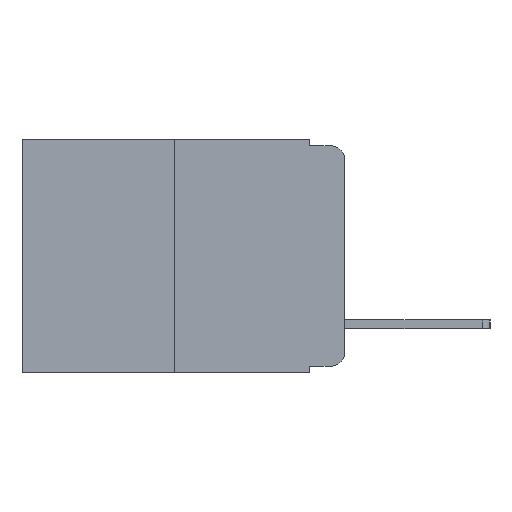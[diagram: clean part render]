
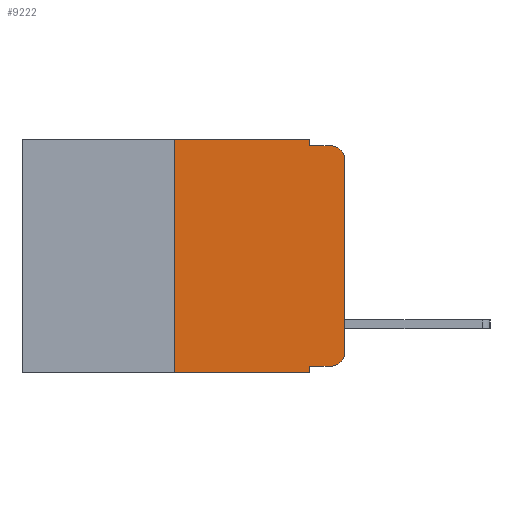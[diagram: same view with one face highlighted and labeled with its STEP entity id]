
A CAD part, left-side view. The second image highlights one B-rep face of the part: STEP entity #9222.
In plain terms, the highlighted planar face has unit normal (-1, 0, 0).
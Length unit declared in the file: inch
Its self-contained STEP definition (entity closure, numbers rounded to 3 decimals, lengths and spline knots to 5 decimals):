
#8 = VECTOR ( 'NONE', #17643, 39.37008 ) ;
#455 = AXIS2_PLACEMENT_3D ( 'NONE', #5341, #14909, #6776 ) ;
#684 = LINE ( 'NONE', #1124, #8795 ) ;
#1057 = CARTESIAN_POINT ( 'NONE',  ( 0., 0.25, -0.343 ) ) ;
#1124 = CARTESIAN_POINT ( 'NONE',  ( 0., 0.473, -0.343 ) ) ;
#1264 = LINE ( 'NONE', #2691, #8838 ) ;
#1283 = DIRECTION ( 'NONE',  ( -1., 0., 0. ) ) ;
#1792 = VERTEX_POINT ( 'NONE', #10440 ) ;
#1930 = CARTESIAN_POINT ( 'NONE',  ( 0., 0.473, 0. ) ) ;
#2372 = CARTESIAN_POINT ( 'NONE',  ( 0., 0., -0.313 ) ) ;
#2661 = EDGE_CURVE ( 'NONE', #11668, #8437, #17009, .T. ) ;
#2691 = CARTESIAN_POINT ( 'NONE',  ( 0., 0.473, 0. ) ) ;
#2696 = DIRECTION ( 'NONE',  ( 0., -1., 0. ) ) ;
#2711 = EDGE_CURVE ( 'NONE', #8437, #9184, #1264, .T. ) ;
#2780 = ORIENTED_EDGE ( 'NONE', *, *, #2970, .F. ) ;
#2793 = EDGE_LOOP ( 'NONE', ( #5871, #9748, #2780, #6755, #7224, #14451, #4226, #8137, #15234, #8626 ) ) ;
#2970 = EDGE_CURVE ( 'NONE', #14234, #1792, #9717, .T. ) ;
#3218 = CARTESIAN_POINT ( 'NONE',  ( 0., 0.051, -0.333 ) ) ;
#3733 = VERTEX_POINT ( 'NONE', #9283 ) ;
#3873 = VERTEX_POINT ( 'NONE', #2372 ) ;
#4061 = VERTEX_POINT ( 'NONE', #8533 ) ;
#4226 = ORIENTED_EDGE ( 'NONE', *, *, #11190, .T. ) ;
#4663 = CARTESIAN_POINT ( 'NONE',  ( 0., 0.051, -0.01 ) ) ;
#5036 = DIRECTION ( 'NONE',  ( 1., 0., 0. ) ) ;
#5195 = CIRCLE ( 'NONE', #12222, 0.02 ) ;
#5341 = CARTESIAN_POINT ( 'NONE',  ( 0., 0.02, -0.03 ) ) ;
#5871 = ORIENTED_EDGE ( 'NONE', *, *, #13366, .T. ) ;
#6300 = VECTOR ( 'NONE', #11859, 39.37008 ) ;
#6755 = ORIENTED_EDGE ( 'NONE', *, *, #8176, .F. ) ;
#6776 = DIRECTION ( 'NONE',  ( 0., 0., -1. ) ) ;
#6871 = VECTOR ( 'NONE', #8499, 39.37008 ) ;
#6993 = CARTESIAN_POINT ( 'NONE',  ( 0., 0.051, 0. ) ) ;
#7224 = ORIENTED_EDGE ( 'NONE', *, *, #2711, .F. ) ;
#7896 = VERTEX_POINT ( 'NONE', #9131 ) ;
#8137 = ORIENTED_EDGE ( 'NONE', *, *, #9379, .F. ) ;
#8176 = EDGE_CURVE ( 'NONE', #9184, #14234, #17019, .T. ) ;
#8437 = VERTEX_POINT ( 'NONE', #18023 ) ;
#8499 = DIRECTION ( 'NONE',  ( 0., 0., 1. ) ) ;
#8533 = CARTESIAN_POINT ( 'NONE',  ( 0., 0., -0.03 ) ) ;
#8626 = ORIENTED_EDGE ( 'NONE', *, *, #10610, .T. ) ;
#8795 = VECTOR ( 'NONE', #11479, 39.37008 ) ;
#8838 = VECTOR ( 'NONE', #2696, 39.37008 ) ;
#9131 = CARTESIAN_POINT ( 'NONE',  ( 0., 0.02, -0.333 ) ) ;
#9133 = VECTOR ( 'NONE', #15678, 39.37008 ) ;
#9184 = VERTEX_POINT ( 'NONE', #12016 ) ;
#9222 = ADVANCED_FACE ( 'NONE', ( #18064 ), #9402, .F. ) ;
#9283 = CARTESIAN_POINT ( 'NONE',  ( 0., 0.051, -0.333 ) ) ;
#9379 = EDGE_CURVE ( 'NONE', #3733, #11312, #15685, .T. ) ;
#9402 = PLANE ( 'NONE',  #17833 ) ;
#9691 = DIRECTION ( 'NONE',  ( 0., 0., -1. ) ) ;
#9717 = LINE ( 'NONE', #4663, #13243 ) ;
#9748 = ORIENTED_EDGE ( 'NONE', *, *, #9787, .T. ) ;
#9787 = EDGE_CURVE ( 'NONE', #4061, #1792, #11491, .T. ) ;
#10009 = LINE ( 'NONE', #3218, #9133 ) ;
#10265 = CARTESIAN_POINT ( 'NONE',  ( 0., 0.02, -0.313 ) ) ;
#10272 = EDGE_CURVE ( 'NONE', #3733, #7896, #10009, .T. ) ;
#10440 = CARTESIAN_POINT ( 'NONE',  ( 0., 0.02, -0.01 ) ) ;
#10610 = EDGE_CURVE ( 'NONE', #7896, #3873, #5195, .T. ) ;
#10648 = VECTOR ( 'NONE', #9691, 39.37008 ) ;
#10752 = LINE ( 'NONE', #16404, #6871 ) ;
#11190 = EDGE_CURVE ( 'NONE', #11668, #11312, #684, .T. ) ;
#11312 = VERTEX_POINT ( 'NONE', #17970 ) ;
#11479 = DIRECTION ( 'NONE',  ( 0., -1., 0. ) ) ;
#11491 = CIRCLE ( 'NONE', #455, 0.02 ) ;
#11624 = DIRECTION ( 'NONE',  ( 0., 0., -1. ) ) ;
#11668 = VERTEX_POINT ( 'NONE', #1057 ) ;
#11700 = CARTESIAN_POINT ( 'NONE',  ( 0., 0.25, 0. ) ) ;
#11859 = DIRECTION ( 'NONE',  ( 0., 0., 1. ) ) ;
#12016 = CARTESIAN_POINT ( 'NONE',  ( 0., 0.051, 0. ) ) ;
#12222 = AXIS2_PLACEMENT_3D ( 'NONE', #10265, #1283, #11624 ) ;
#13243 = VECTOR ( 'NONE', #16444, 39.37008 ) ;
#13366 = EDGE_CURVE ( 'NONE', #3873, #4061, #10752, .T. ) ;
#14234 = VERTEX_POINT ( 'NONE', #16058 ) ;
#14451 = ORIENTED_EDGE ( 'NONE', *, *, #2661, .F. ) ;
#14667 = DIRECTION ( 'NONE',  ( 0., 0., -1. ) ) ;
#14909 = DIRECTION ( 'NONE',  ( -1., 0., 0. ) ) ;
#15234 = ORIENTED_EDGE ( 'NONE', *, *, #10272, .T. ) ;
#15678 = DIRECTION ( 'NONE',  ( 0., -1., 0. ) ) ;
#15685 = LINE ( 'NONE', #6993, #8 ) ;
#16058 = CARTESIAN_POINT ( 'NONE',  ( 0., 0.051, -0.01 ) ) ;
#16404 = CARTESIAN_POINT ( 'NONE',  ( 0., 0., 0. ) ) ;
#16444 = DIRECTION ( 'NONE',  ( 0., -1., 0. ) ) ;
#17009 = LINE ( 'NONE', #11700, #6300 ) ;
#17019 = LINE ( 'NONE', #17406, #10648 ) ;
#17406 = CARTESIAN_POINT ( 'NONE',  ( 0., 0.051, 0. ) ) ;
#17643 = DIRECTION ( 'NONE',  ( 0., 0., -1. ) ) ;
#17833 = AXIS2_PLACEMENT_3D ( 'NONE', #1930, #5036, #14667 ) ;
#17970 = CARTESIAN_POINT ( 'NONE',  ( 0., 0.051, -0.343 ) ) ;
#18023 = CARTESIAN_POINT ( 'NONE',  ( 0., 0.25, 0. ) ) ;
#18064 = FACE_OUTER_BOUND ( 'NONE', #2793, .T. ) ;
